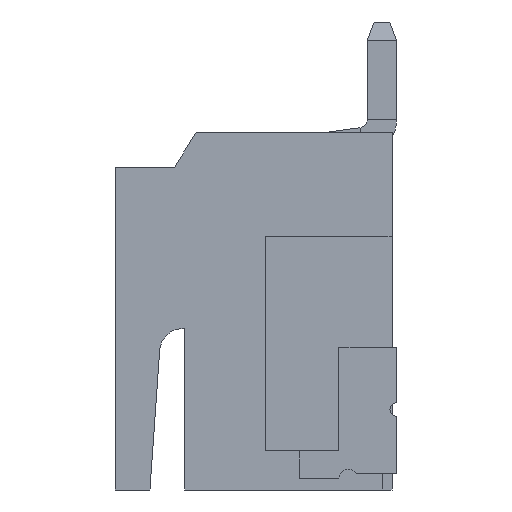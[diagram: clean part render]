
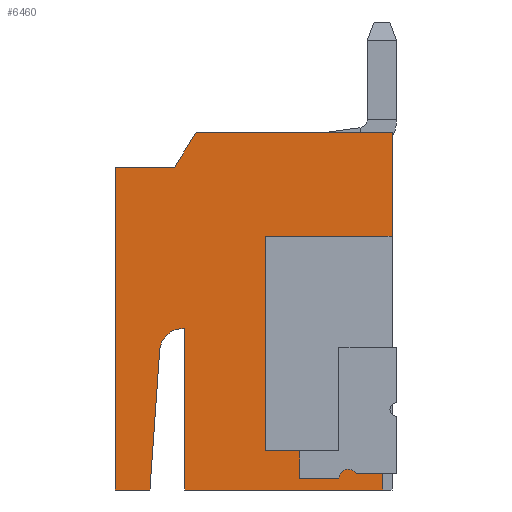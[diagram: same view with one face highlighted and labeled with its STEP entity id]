
A CAD part, left-side view. The second image highlights one B-rep face of the part: STEP entity #6460.
In plain terms, the highlighted planar face has unit normal (-1, 0, 0).
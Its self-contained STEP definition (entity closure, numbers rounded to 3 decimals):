
#46 = VECTOR ( 'NONE', #6970, 1000. ) ;
#153 = LINE ( 'NONE', #2012, #6529 ) ;
#243 = VERTEX_POINT ( 'NONE', #1535 ) ;
#268 = CARTESIAN_POINT ( 'NONE',  ( -8.75, 1.439, -0.873 ) ) ;
#303 = CARTESIAN_POINT ( 'NONE',  ( -8.75, -3.1, 3.875 ) ) ;
#434 = CIRCLE ( 'NONE', #4913, 0.5 ) ;
#560 = ORIENTED_EDGE ( 'NONE', *, *, #6510, .F. ) ;
#667 = EDGE_CURVE ( 'NONE', #2687, #7352, #881, .T. ) ;
#683 = VECTOR ( 'NONE', #1773, 1000. ) ;
#794 = ORIENTED_EDGE ( 'NONE', *, *, #4077, .F. ) ;
#798 = LINE ( 'NONE', #7379, #7550 ) ;
#810 = VECTOR ( 'NONE', #7810, 1000. ) ;
#867 = CARTESIAN_POINT ( 'NONE',  ( -8.75, 1.4, -3.875 ) ) ;
#868 = CARTESIAN_POINT ( 'NONE',  ( -8.75, -2.15, -3.625 ) ) ;
#881 = LINE ( 'NONE', #2209, #2448 ) ;
#946 = CARTESIAN_POINT ( 'NONE',  ( -8.75, 1.938, -0.839 ) ) ;
#948 = VECTOR ( 'NONE', #4278, 1000. ) ;
#957 = ORIENTED_EDGE ( 'NONE', *, *, #2039, .F. ) ;
#995 = EDGE_CURVE ( 'NONE', #6064, #1186, #7363, .T. ) ;
#1119 = AXIS2_PLACEMENT_3D ( 'NONE', #2395, #3670, #3074 ) ;
#1166 = EDGE_CURVE ( 'NONE', #3169, #5983, #6293, .T. ) ;
#1186 = VERTEX_POINT ( 'NONE', #946 ) ;
#1203 = CARTESIAN_POINT ( 'NONE',  ( -8.75, 1.619, 3.125 ) ) ;
#1211 = CARTESIAN_POINT ( 'NONE',  ( -8.75, -2.9, 1.625 ) ) ;
#1229 = ORIENTED_EDGE ( 'NONE', *, *, #7728, .T. ) ;
#1463 = VERTEX_POINT ( 'NONE', #3713 ) ;
#1483 = CARTESIAN_POINT ( 'NONE',  ( -8.75, 1.4, -0.375 ) ) ;
#1500 = VECTOR ( 'NONE', #7330, 1000. ) ;
#1501 = DIRECTION ( 'NONE',  ( 0., -1., 0. ) ) ;
#1535 = CARTESIAN_POINT ( 'NONE',  ( -8.75, 2.9, 3.125 ) ) ;
#1639 = EDGE_CURVE ( 'NONE', #243, #7631, #4762, .T. ) ;
#1644 = CARTESIAN_POINT ( 'NONE',  ( -8.75, 2.9, 3.125 ) ) ;
#1688 = CARTESIAN_POINT ( 'NONE',  ( -8.75, -1.1, -3.625 ) ) ;
#1773 = DIRECTION ( 'NONE',  ( 0., -1., 0. ) ) ;
#1981 = LINE ( 'NONE', #4421, #4935 ) ;
#1992 = DIRECTION ( 'NONE',  ( -1., 0., 0. ) ) ;
#2005 = VERTEX_POINT ( 'NONE', #3642 ) ;
#2012 = CARTESIAN_POINT ( 'NONE',  ( -8.75, 2.9, -3.875 ) ) ;
#2039 = EDGE_CURVE ( 'NONE', #7631, #1463, #7325, .T. ) ;
#2067 = VERTEX_POINT ( 'NONE', #5024 ) ;
#2115 = ORIENTED_EDGE ( 'NONE', *, *, #2153, .T. ) ;
#2117 = LINE ( 'NONE', #4548, #46 ) ;
#2123 = CARTESIAN_POINT ( 'NONE',  ( -8.75, 1.4, 0. ) ) ;
#2153 = EDGE_CURVE ( 'NONE', #4320, #5087, #6053, .T. ) ;
#2189 = EDGE_CURVE ( 'NONE', #6244, #6406, #2117, .T. ) ;
#2209 = CARTESIAN_POINT ( 'NONE',  ( -8.75, -2.9, -3.875 ) ) ;
#2357 = LINE ( 'NONE', #7166, #6893 ) ;
#2375 = DIRECTION ( 'NONE',  ( 0., 1., 0. ) ) ;
#2395 = CARTESIAN_POINT ( 'NONE',  ( -8.75, 0., 0. ) ) ;
#2448 = VECTOR ( 'NONE', #3963, 1000. ) ;
#2637 = VECTOR ( 'NONE', #6146, 1000. ) ;
#2681 = VECTOR ( 'NONE', #7175, 1000. ) ;
#2687 = VERTEX_POINT ( 'NONE', #5813 ) ;
#2755 = CARTESIAN_POINT ( 'NONE',  ( -8.75, 2.15, -3.875 ) ) ;
#2761 = DIRECTION ( 'NONE',  ( 0., 0., 1. ) ) ;
#2830 = ORIENTED_EDGE ( 'NONE', *, *, #6912, .T. ) ;
#2873 = CARTESIAN_POINT ( 'NONE',  ( -8.75, -1.1, -3.625 ) ) ;
#2886 = ORIENTED_EDGE ( 'NONE', *, *, #7232, .F. ) ;
#2980 = LINE ( 'NONE', #1211, #683 ) ;
#2992 = ORIENTED_EDGE ( 'NONE', *, *, #2189, .T. ) ;
#3016 = VECTOR ( 'NONE', #4513, 1000. ) ;
#3051 = VERTEX_POINT ( 'NONE', #4412 ) ;
#3074 = DIRECTION ( 'NONE',  ( 0., 0., -1. ) ) ;
#3169 = VERTEX_POINT ( 'NONE', #5326 ) ;
#3419 = CARTESIAN_POINT ( 'NONE',  ( -8.75, 1.619, 3.125 ) ) ;
#3498 = ORIENTED_EDGE ( 'NONE', *, *, #7289, .T. ) ;
#3538 = EDGE_CURVE ( 'NONE', #6064, #3539, #2357, .T. ) ;
#3539 = VERTEX_POINT ( 'NONE', #7708 ) ;
#3612 = VERTEX_POINT ( 'NONE', #1483 ) ;
#3639 = CARTESIAN_POINT ( 'NONE',  ( -8.75, -3.1, 3.875 ) ) ;
#3642 = CARTESIAN_POINT ( 'NONE',  ( -8.75, -2.9, -3.525 ) ) ;
#3670 = DIRECTION ( 'NONE',  ( 1., 0., 0. ) ) ;
#3713 = CARTESIAN_POINT ( 'NONE',  ( -8.75, 1.15, 3.875 ) ) ;
#3818 = ORIENTED_EDGE ( 'NONE', *, *, #995, .T. ) ;
#3867 = DIRECTION ( 'NONE',  ( 0., 0., -1. ) ) ;
#3963 = DIRECTION ( 'NONE',  ( 0., 1., 0. ) ) ;
#4077 = EDGE_CURVE ( 'NONE', #3539, #243, #153, .T. ) ;
#4196 = DIRECTION ( 'NONE',  ( 0., 1., 0. ) ) ;
#4278 = DIRECTION ( 'NONE',  ( 0., -0.53, 0.848 ) ) ;
#4320 = VERTEX_POINT ( 'NONE', #5482 ) ;
#4412 = CARTESIAN_POINT ( 'NONE',  ( -8.75, -0.35, -3.025 ) ) ;
#4421 = CARTESIAN_POINT ( 'NONE',  ( -8.75, 1.15, 3.875 ) ) ;
#4442 = EDGE_LOOP ( 'NONE', ( #4716, #1229, #6750, #2886, #5490, #2115, #7050, #2992, #5111, #2830, #3498, #6493, #560, #957, #7057, #794, #6221, #3818 ) ) ;
#4513 = DIRECTION ( 'NONE',  ( 0., 0., -1. ) ) ;
#4548 = CARTESIAN_POINT ( 'NONE',  ( -8.75, -1.1, -0.775 ) ) ;
#4716 = ORIENTED_EDGE ( 'NONE', *, *, #7804, .T. ) ;
#4762 = LINE ( 'NONE', #1644, #2681 ) ;
#4913 = AXIS2_PLACEMENT_3D ( 'NONE', #268, #5237, #6628 ) ;
#4935 = VECTOR ( 'NONE', #1501, 1000. ) ;
#4969 = DIRECTION ( 'NONE',  ( 0., 0., 1. ) ) ;
#5004 = VECTOR ( 'NONE', #2761, 1000. ) ;
#5024 = CARTESIAN_POINT ( 'NONE',  ( -8.75, -0.35, 1.625 ) ) ;
#5087 = VERTEX_POINT ( 'NONE', #7745 ) ;
#5097 = EDGE_CURVE ( 'NONE', #2005, #4320, #5858, .T. ) ;
#5111 = ORIENTED_EDGE ( 'NONE', *, *, #5589, .T. ) ;
#5237 = DIRECTION ( 'NONE',  ( 1., 0., 0. ) ) ;
#5292 = VECTOR ( 'NONE', #2375, 1000. ) ;
#5314 = VECTOR ( 'NONE', #5819, 1000. ) ;
#5326 = CARTESIAN_POINT ( 'NONE',  ( -8.75, -3.1, 1.625 ) ) ;
#5443 = CARTESIAN_POINT ( 'NONE',  ( -8.75, -0.35, -3.025 ) ) ;
#5482 = CARTESIAN_POINT ( 'NONE',  ( -8.75, -2.323, -3.525 ) ) ;
#5490 = ORIENTED_EDGE ( 'NONE', *, *, #5097, .T. ) ;
#5589 = EDGE_CURVE ( 'NONE', #6406, #3051, #6674, .T. ) ;
#5813 = CARTESIAN_POINT ( 'NONE',  ( -8.75, -2.9, -3.875 ) ) ;
#5819 = DIRECTION ( 'NONE',  ( 0., 1., 0. ) ) ;
#5858 = LINE ( 'NONE', #6449, #5314 ) ;
#5961 = LINE ( 'NONE', #6222, #810 ) ;
#5983 = VERTEX_POINT ( 'NONE', #3639 ) ;
#6053 = CIRCLE ( 'NONE', #7551, 0.2 ) ;
#6058 = CARTESIAN_POINT ( 'NONE',  ( -8.75, -1.1, -3.025 ) ) ;
#6064 = VERTEX_POINT ( 'NONE', #2755 ) ;
#6146 = DIRECTION ( 'NONE',  ( 0., -0.07, 0.998 ) ) ;
#6221 = ORIENTED_EDGE ( 'NONE', *, *, #3538, .F. ) ;
#6222 = CARTESIAN_POINT ( 'NONE',  ( -8.75, -2.9, 3.875 ) ) ;
#6244 = VERTEX_POINT ( 'NONE', #2873 ) ;
#6293 = LINE ( 'NONE', #303, #5004 ) ;
#6406 = VERTEX_POINT ( 'NONE', #6058 ) ;
#6449 = CARTESIAN_POINT ( 'NONE',  ( -8.75, -2.323, -3.525 ) ) ;
#6460 = ADVANCED_FACE ( 'NONE', ( #7351 ), #6692, .F. ) ;
#6493 = ORIENTED_EDGE ( 'NONE', *, *, #1166, .T. ) ;
#6510 = EDGE_CURVE ( 'NONE', #1463, #5983, #1981, .T. ) ;
#6529 = VECTOR ( 'NONE', #6986, 1000. ) ;
#6628 = DIRECTION ( 'NONE',  ( 0., 0., -1. ) ) ;
#6674 = LINE ( 'NONE', #5443, #1500 ) ;
#6692 = PLANE ( 'NONE',  #1119 ) ;
#6750 = ORIENTED_EDGE ( 'NONE', *, *, #667, .F. ) ;
#6814 = LINE ( 'NONE', #1688, #5292 ) ;
#6893 = VECTOR ( 'NONE', #4196, 1000. ) ;
#6912 = EDGE_CURVE ( 'NONE', #3051, #2067, #798, .T. ) ;
#6970 = DIRECTION ( 'NONE',  ( 0., 0., 1. ) ) ;
#6977 = LINE ( 'NONE', #2123, #3016 ) ;
#6986 = DIRECTION ( 'NONE',  ( 0., 0., 1. ) ) ;
#7050 = ORIENTED_EDGE ( 'NONE', *, *, #7198, .T. ) ;
#7057 = ORIENTED_EDGE ( 'NONE', *, *, #1639, .F. ) ;
#7166 = CARTESIAN_POINT ( 'NONE',  ( -8.75, -2.9, -3.875 ) ) ;
#7175 = DIRECTION ( 'NONE',  ( 0., -1., 0. ) ) ;
#7198 = EDGE_CURVE ( 'NONE', #5087, #6244, #6814, .T. ) ;
#7232 = EDGE_CURVE ( 'NONE', #2005, #2687, #5961, .T. ) ;
#7288 = CARTESIAN_POINT ( 'NONE',  ( -8.75, 1.87, 0.131 ) ) ;
#7289 = EDGE_CURVE ( 'NONE', #2067, #3169, #2980, .T. ) ;
#7325 = LINE ( 'NONE', #1203, #948 ) ;
#7330 = DIRECTION ( 'NONE',  ( 0., 1., 0. ) ) ;
#7351 = FACE_OUTER_BOUND ( 'NONE', #4442, .T. ) ;
#7352 = VERTEX_POINT ( 'NONE', #867 ) ;
#7363 = LINE ( 'NONE', #7288, #2637 ) ;
#7379 = CARTESIAN_POINT ( 'NONE',  ( -8.75, -0.35, 1.625 ) ) ;
#7550 = VECTOR ( 'NONE', #4969, 1000. ) ;
#7551 = AXIS2_PLACEMENT_3D ( 'NONE', #868, #1992, #3867 ) ;
#7631 = VERTEX_POINT ( 'NONE', #3419 ) ;
#7708 = CARTESIAN_POINT ( 'NONE',  ( -8.75, 2.9, -3.875 ) ) ;
#7728 = EDGE_CURVE ( 'NONE', #3612, #7352, #6977, .T. ) ;
#7745 = CARTESIAN_POINT ( 'NONE',  ( -8.75, -1.95, -3.625 ) ) ;
#7804 = EDGE_CURVE ( 'NONE', #1186, #3612, #434, .T. ) ;
#7810 = DIRECTION ( 'NONE',  ( 0., 0., -1. ) ) ;
